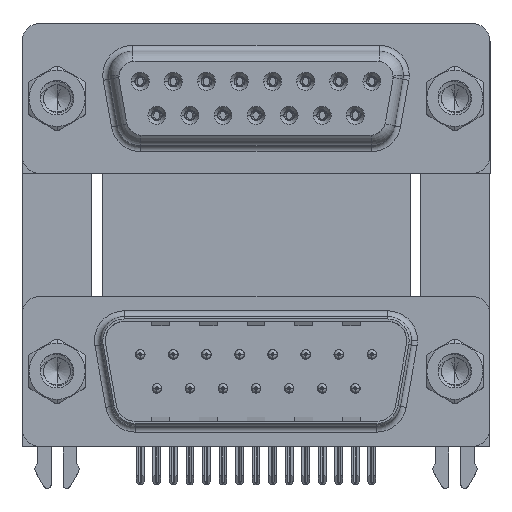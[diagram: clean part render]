
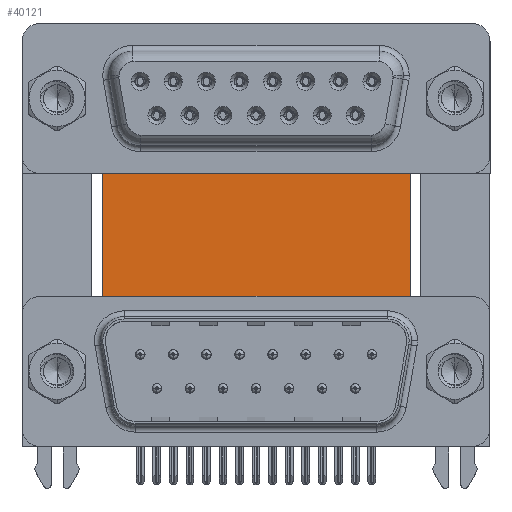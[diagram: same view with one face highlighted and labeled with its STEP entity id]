
A CAD part, top view. The second image highlights one B-rep face of the part: STEP entity #40121.
In plain terms, the highlighted planar face has unit normal (0, 0, 1).
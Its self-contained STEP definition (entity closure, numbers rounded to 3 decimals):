
#1632 = LINE ( 'NONE', #17018, #7118 ) ;
#5767 = LINE ( 'NONE', #45840, #30523 ) ;
#6318 = EDGE_CURVE ( 'NONE', #38607, #19699, #10963, .T. ) ;
#7118 = VECTOR ( 'NONE', #45366, 1000. ) ;
#7511 = ORIENTED_EDGE ( 'NONE', *, *, #21199, .F. ) ;
#8517 = VECTOR ( 'NONE', #8682, 1000. ) ;
#8682 = DIRECTION ( 'NONE',  ( 0., -1., 0. ) ) ;
#10963 = LINE ( 'NONE', #51294, #36026 ) ;
#11622 = CARTESIAN_POINT ( 'NONE',  ( 29.58, 16.585, -12. ) ) ;
#12438 = ORIENTED_EDGE ( 'NONE', *, *, #50503, .T. ) ;
#17018 = CARTESIAN_POINT ( 'NONE',  ( 3.79, -3.735, -12. ) ) ;
#17502 = DIRECTION ( 'NONE',  ( 0., -1., 0. ) ) ;
#19699 = VERTEX_POINT ( 'NONE', #11622 ) ;
#19991 = CARTESIAN_POINT ( 'NONE',  ( 3.79, 16.585, -12. ) ) ;
#20654 = CARTESIAN_POINT ( 'NONE',  ( 29.58, 16.585, -12. ) ) ;
#21199 = EDGE_CURVE ( 'NONE', #19699, #36060, #44350, .T. ) ;
#21605 = VERTEX_POINT ( 'NONE', #50753 ) ;
#30308 = PLANE ( 'NONE',  #43083 ) ;
#30523 = VECTOR ( 'NONE', #17502, 1000. ) ;
#31166 = ORIENTED_EDGE ( 'NONE', *, *, #6318, .F. ) ;
#33736 = CARTESIAN_POINT ( 'NONE',  ( 3.79, 16.585, -12. ) ) ;
#36026 = VECTOR ( 'NONE', #50785, 1000. ) ;
#36060 = VERTEX_POINT ( 'NONE', #46272 ) ;
#36897 = EDGE_CURVE ( 'NONE', #38607, #21605, #5767, .T. ) ;
#38607 = VERTEX_POINT ( 'NONE', #19991 ) ;
#40121 = ADVANCED_FACE ( 'NONE', ( #42051 ), #30308, .F. ) ;
#41027 = DIRECTION ( 'NONE',  ( 0., 0., -1. ) ) ;
#41958 = ORIENTED_EDGE ( 'NONE', *, *, #36897, .T. ) ;
#42051 = FACE_OUTER_BOUND ( 'NONE', #48256, .T. ) ;
#43083 = AXIS2_PLACEMENT_3D ( 'NONE', #33736, #41027, #49078 ) ;
#44350 = LINE ( 'NONE', #20654, #8517 ) ;
#45366 = DIRECTION ( 'NONE',  ( 1., 0., 0. ) ) ;
#45840 = CARTESIAN_POINT ( 'NONE',  ( 3.79, 16.585, -12. ) ) ;
#46272 = CARTESIAN_POINT ( 'NONE',  ( 29.58, -3.735, -12. ) ) ;
#48256 = EDGE_LOOP ( 'NONE', ( #12438, #7511, #31166, #41958 ) ) ;
#49078 = DIRECTION ( 'NONE',  ( -1., 0., 0. ) ) ;
#50503 = EDGE_CURVE ( 'NONE', #21605, #36060, #1632, .T. ) ;
#50753 = CARTESIAN_POINT ( 'NONE',  ( 3.79, -3.735, -12. ) ) ;
#50785 = DIRECTION ( 'NONE',  ( 1., 0., 0. ) ) ;
#51294 = CARTESIAN_POINT ( 'NONE',  ( 3.79, 16.585, -12. ) ) ;
